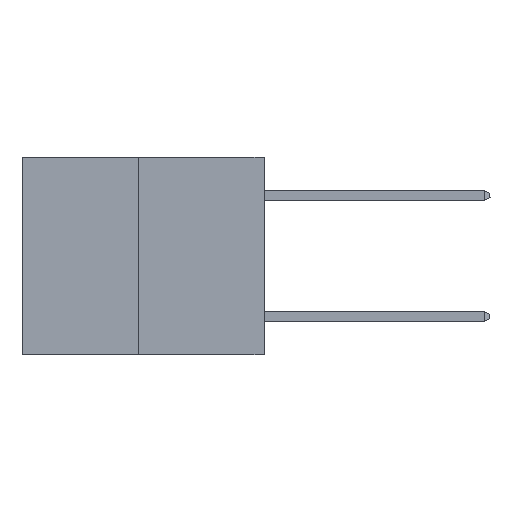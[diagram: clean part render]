
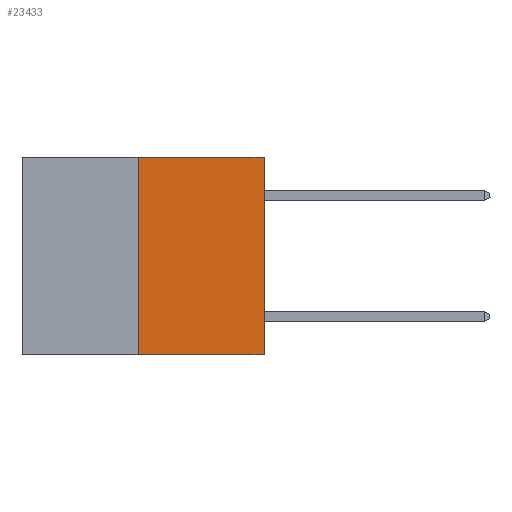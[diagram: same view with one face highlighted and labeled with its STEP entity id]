
A CAD part, left-side view. The second image highlights one B-rep face of the part: STEP entity #23433.
In plain terms, the highlighted planar face has unit normal (-1, 0, 0).
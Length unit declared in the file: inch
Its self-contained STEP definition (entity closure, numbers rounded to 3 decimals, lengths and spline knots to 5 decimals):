
#1236 = LINE ( 'NONE', #18793, #20007 ) ;
#1378 = ORIENTED_EDGE ( 'NONE', *, *, #19398, .F. ) ;
#2955 = CARTESIAN_POINT ( 'NONE',  ( 0., 0., 0. ) ) ;
#3316 = CARTESIAN_POINT ( 'NONE',  ( 0., 0.6, 0. ) ) ;
#6991 = EDGE_CURVE ( 'NONE', #27513, #25811, #20765, .T. ) ;
#7714 = VECTOR ( 'NONE', #26715, 39.37008 ) ;
#9176 = PLANE ( 'NONE',  #28947 ) ;
#9767 = CARTESIAN_POINT ( 'NONE',  ( 0., 0.312, -0.49 ) ) ;
#10088 = DIRECTION ( 'NONE',  ( 0., 0., 1. ) ) ;
#11000 = CARTESIAN_POINT ( 'NONE',  ( 0., 0., 0. ) ) ;
#11817 = EDGE_LOOP ( 'NONE', ( #1378, #16722, #24245, #12934 ) ) ;
#12934 = ORIENTED_EDGE ( 'NONE', *, *, #16054, .F. ) ;
#13596 = DIRECTION ( 'NONE',  ( 0., -1., 0. ) ) ;
#14215 = VERTEX_POINT ( 'NONE', #21144 ) ;
#14479 = DIRECTION ( 'NONE',  ( 0., 0., 1. ) ) ;
#14548 = DIRECTION ( 'NONE',  ( 0., 0., -1. ) ) ;
#14651 = EDGE_CURVE ( 'NONE', #25811, #16117, #19475, .T. ) ;
#14755 = VECTOR ( 'NONE', #13596, 39.37008 ) ;
#16054 = EDGE_CURVE ( 'NONE', #14215, #16117, #28224, .T. ) ;
#16117 = VERTEX_POINT ( 'NONE', #11000 ) ;
#16722 = ORIENTED_EDGE ( 'NONE', *, *, #6991, .T. ) ;
#17114 = CARTESIAN_POINT ( 'NONE',  ( 0., 0., -0.49 ) ) ;
#18793 = CARTESIAN_POINT ( 'NONE',  ( 0., 0.312, -0.49 ) ) ;
#19158 = DIRECTION ( 'NONE',  ( 1., 0., 0. ) ) ;
#19398 = EDGE_CURVE ( 'NONE', #27513, #14215, #1236, .T. ) ;
#19475 = LINE ( 'NONE', #2955, #25857 ) ;
#20007 = VECTOR ( 'NONE', #14479, 39.37008 ) ;
#20765 = LINE ( 'NONE', #22701, #14755 ) ;
#21144 = CARTESIAN_POINT ( 'NONE',  ( 0., 0.312, 0. ) ) ;
#22701 = CARTESIAN_POINT ( 'NONE',  ( 0., 0.6, -0.49 ) ) ;
#23433 = ADVANCED_FACE ( 'NONE', ( #28539 ), #9176, .F. ) ;
#24245 = ORIENTED_EDGE ( 'NONE', *, *, #14651, .T. ) ;
#25811 = VERTEX_POINT ( 'NONE', #17114 ) ;
#25857 = VECTOR ( 'NONE', #10088, 39.37008 ) ;
#26715 = DIRECTION ( 'NONE',  ( 0., -1., 0. ) ) ;
#27513 = VERTEX_POINT ( 'NONE', #9767 ) ;
#28224 = LINE ( 'NONE', #28499, #7714 ) ;
#28499 = CARTESIAN_POINT ( 'NONE',  ( 0., 0.6, 0. ) ) ;
#28539 = FACE_OUTER_BOUND ( 'NONE', #11817, .T. ) ;
#28947 = AXIS2_PLACEMENT_3D ( 'NONE', #3316, #19158, #14548 ) ;
